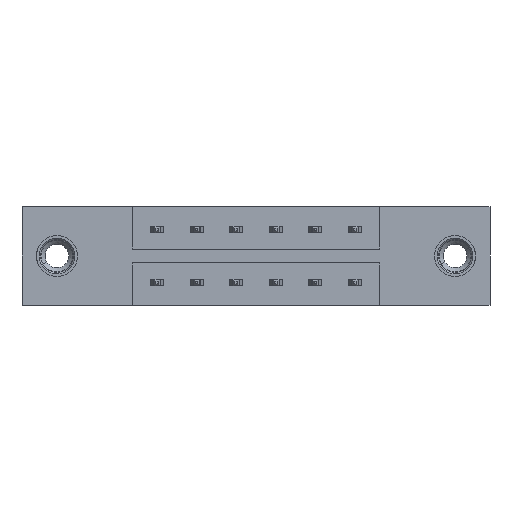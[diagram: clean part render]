
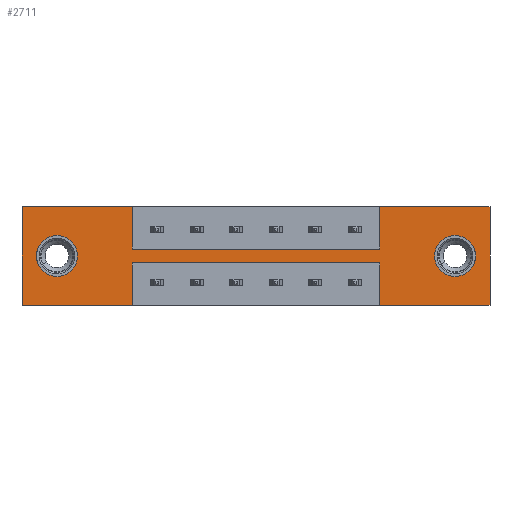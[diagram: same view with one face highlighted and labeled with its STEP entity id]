
A CAD part, front view. The second image highlights one B-rep face of the part: STEP entity #2711.
In plain terms, the highlighted planar face has unit normal (0, -1, 0).
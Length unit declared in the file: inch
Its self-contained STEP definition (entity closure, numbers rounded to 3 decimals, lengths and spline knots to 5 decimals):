
#9 = ORIENTED_EDGE ( 'NONE', *, *, #3987, .F. ) ;
#28 = CARTESIAN_POINT ( 'NONE',  ( 0.1325, 0., -0.1095 ) ) ;
#43 = AXIS2_PLACEMENT_3D ( 'NONE', #4647, #4583, #858 ) ;
#75 = VERTEX_POINT ( 'NONE', #8183 ) ;
#105 = EDGE_CURVE ( 'NONE', #1922, #75, #3162, .T. ) ;
#159 = EDGE_CURVE ( 'NONE', #5463, #1922, #8088, .T. ) ;
#179 = DIRECTION ( 'NONE',  ( 0., 0., -1. ) ) ;
#241 = VERTEX_POINT ( 'NONE', #5210 ) ;
#253 = DIRECTION ( 'NONE',  ( 0., 0., -1. ) ) ;
#374 = VERTEX_POINT ( 'NONE', #9278 ) ;
#519 = LINE ( 'NONE', #8531, #4059 ) ;
#583 = DIRECTION ( 'NONE',  ( 0., 0., 1. ) ) ;
#628 = FACE_BOUND ( 'NONE', #6813, .T. ) ;
#663 = VECTOR ( 'NONE', #9193, 39.37008 ) ;
#706 = EDGE_LOOP ( 'NONE', ( #8567, #3923 ) ) ;
#814 = CARTESIAN_POINT ( 'NONE',  ( 1.3575, 0., -0.161 ) ) ;
#851 = CARTESIAN_POINT ( 'NONE',  ( 0., 0., -0.375 ) ) ;
#858 = DIRECTION ( 'NONE',  ( 0., 0., -1. ) ) ;
#913 = ORIENTED_EDGE ( 'NONE', *, *, #3880, .F. ) ;
#954 = EDGE_CURVE ( 'NONE', #241, #374, #7257, .T. ) ;
#984 = CARTESIAN_POINT ( 'NONE',  ( 0., 0., -0.375 ) ) ;
#1067 = ORIENTED_EDGE ( 'NONE', *, *, #5295, .T. ) ;
#1130 = VECTOR ( 'NONE', #2078, 39.37008 ) ;
#1239 = EDGE_CURVE ( 'NONE', #5102, #2460, #4670, .T. ) ;
#1309 = CARTESIAN_POINT ( 'NONE',  ( 0.4175, 0., -0.161 ) ) ;
#1341 = CARTESIAN_POINT ( 'NONE',  ( 0., 0., 0. ) ) ;
#1405 = DIRECTION ( 'NONE',  ( 0., 1., 0. ) ) ;
#1406 = VERTEX_POINT ( 'NONE', #3636 ) ;
#1630 = CARTESIAN_POINT ( 'NONE',  ( 1.6425, 0., -0.1875 ) ) ;
#1670 = EDGE_CURVE ( 'NONE', #1406, #6208, #9110, .T. ) ;
#1763 = DIRECTION ( 'NONE',  ( 0., 0., -1. ) ) ;
#1913 = VECTOR ( 'NONE', #2419, 39.37008 ) ;
#1922 = VERTEX_POINT ( 'NONE', #5045 ) ;
#2024 = LINE ( 'NONE', #1309, #6029 ) ;
#2039 = CARTESIAN_POINT ( 'NONE',  ( 0.4175, 0., -0.214 ) ) ;
#2078 = DIRECTION ( 'NONE',  ( 1., 0., 0. ) ) ;
#2124 = EDGE_CURVE ( 'NONE', #374, #241, #6973, .T. ) ;
#2221 = VECTOR ( 'NONE', #8911, 39.37008 ) ;
#2318 = DIRECTION ( 'NONE',  ( 0., 0., 1. ) ) ;
#2326 = LINE ( 'NONE', #5393, #3517 ) ;
#2419 = DIRECTION ( 'NONE',  ( 0., 0., 1. ) ) ;
#2433 = DIRECTION ( 'NONE',  ( 1., 0., 0. ) ) ;
#2460 = VERTEX_POINT ( 'NONE', #9529 ) ;
#2687 = CARTESIAN_POINT ( 'NONE',  ( 1.3575, 0., -0.161 ) ) ;
#2711 = ADVANCED_FACE ( 'NONE', ( #6384, #628, #5810 ), #6848, .T. ) ;
#2805 = EDGE_CURVE ( 'NONE', #6142, #5102, #4406, .T. ) ;
#2875 = CARTESIAN_POINT ( 'NONE',  ( 0.1325, 0., -0.1875 ) ) ;
#2885 = ORIENTED_EDGE ( 'NONE', *, *, #1239, .F. ) ;
#2954 = EDGE_CURVE ( 'NONE', #7374, #1406, #519, .T. ) ;
#3088 = DIRECTION ( 'NONE',  ( 0., -1., 0. ) ) ;
#3132 = EDGE_CURVE ( 'NONE', #2460, #4090, #2024, .T. ) ;
#3162 = LINE ( 'NONE', #9605, #2221 ) ;
#3517 = VECTOR ( 'NONE', #2433, 39.37008 ) ;
#3620 = CIRCLE ( 'NONE', #6883, 0.078 ) ;
#3636 = CARTESIAN_POINT ( 'NONE',  ( 1.775, 0., -0.375 ) ) ;
#3832 = CARTESIAN_POINT ( 'NONE',  ( 1.775, 0., 0. ) ) ;
#3880 = EDGE_CURVE ( 'NONE', #6208, #5463, #4092, .T. ) ;
#3923 = ORIENTED_EDGE ( 'NONE', *, *, #2124, .T. ) ;
#3987 = EDGE_CURVE ( 'NONE', #75, #6142, #4557, .T. ) ;
#4059 = VECTOR ( 'NONE', #1763, 39.37008 ) ;
#4090 = VERTEX_POINT ( 'NONE', #4901 ) ;
#4092 = LINE ( 'NONE', #8894, #7470 ) ;
#4104 = VERTEX_POINT ( 'NONE', #2687 ) ;
#4259 = ORIENTED_EDGE ( 'NONE', *, *, #2954, .F. ) ;
#4289 = ORIENTED_EDGE ( 'NONE', *, *, #2805, .F. ) ;
#4406 = LINE ( 'NONE', #8373, #1913 ) ;
#4555 = EDGE_LOOP ( 'NONE', ( #913, #6363, #4259, #5035, #7524, #6803, #5549, #2885, #4289, #9, #8755, #8306 ) ) ;
#4557 = LINE ( 'NONE', #984, #663 ) ;
#4583 = DIRECTION ( 'NONE',  ( 0., 1., 0. ) ) ;
#4647 = CARTESIAN_POINT ( 'NONE',  ( 1.6425, 0., -0.1875 ) ) ;
#4653 = CARTESIAN_POINT ( 'NONE',  ( 1.3575, 0., -0.375 ) ) ;
#4670 = LINE ( 'NONE', #1341, #1130 ) ;
#4729 = VERTEX_POINT ( 'NONE', #28 ) ;
#4767 = DIRECTION ( 'NONE',  ( 0., 1., 0. ) ) ;
#4894 = CARTESIAN_POINT ( 'NONE',  ( 0., 0., -0.375 ) ) ;
#4901 = CARTESIAN_POINT ( 'NONE',  ( 0.4175, 0., -0.161 ) ) ;
#4979 = CARTESIAN_POINT ( 'NONE',  ( 0., 0., 0. ) ) ;
#5000 = DIRECTION ( 'NONE',  ( 0., 1., 0. ) ) ;
#5035 = ORIENTED_EDGE ( 'NONE', *, *, #5104, .F. ) ;
#5045 = CARTESIAN_POINT ( 'NONE',  ( 0.4175, 0., -0.214 ) ) ;
#5102 = VERTEX_POINT ( 'NONE', #4979 ) ;
#5104 = EDGE_CURVE ( 'NONE', #6469, #7374, #9489, .T. ) ;
#5210 = CARTESIAN_POINT ( 'NONE',  ( 1.6425, 0., -0.1095 ) ) ;
#5295 = EDGE_CURVE ( 'NONE', #4729, #8133, #3620, .T. ) ;
#5393 = CARTESIAN_POINT ( 'NONE',  ( 0.4175, 0., -0.161 ) ) ;
#5463 = VERTEX_POINT ( 'NONE', #8370 ) ;
#5501 = VECTOR ( 'NONE', #7284, 39.37008 ) ;
#5549 = ORIENTED_EDGE ( 'NONE', *, *, #3132, .F. ) ;
#5810 = FACE_OUTER_BOUND ( 'NONE', #4555, .T. ) ;
#6029 = VECTOR ( 'NONE', #7369, 39.37008 ) ;
#6072 = LINE ( 'NONE', #814, #6437 ) ;
#6142 = VERTEX_POINT ( 'NONE', #4894 ) ;
#6208 = VERTEX_POINT ( 'NONE', #4653 ) ;
#6363 = ORIENTED_EDGE ( 'NONE', *, *, #1670, .F. ) ;
#6384 = FACE_BOUND ( 'NONE', #706, .T. ) ;
#6437 = VECTOR ( 'NONE', #2318, 39.37008 ) ;
#6469 = VERTEX_POINT ( 'NONE', #8650 ) ;
#6643 = DIRECTION ( 'NONE',  ( -1., 0., 0. ) ) ;
#6648 = ORIENTED_EDGE ( 'NONE', *, *, #8028, .T. ) ;
#6769 = AXIS2_PLACEMENT_3D ( 'NONE', #2875, #5000, #583 ) ;
#6803 = ORIENTED_EDGE ( 'NONE', *, *, #9226, .F. ) ;
#6813 = EDGE_LOOP ( 'NONE', ( #1067, #6648 ) ) ;
#6848 = PLANE ( 'NONE',  #8982 ) ;
#6883 = AXIS2_PLACEMENT_3D ( 'NONE', #8143, #1405, #8065 ) ;
#6907 = CIRCLE ( 'NONE', #6769, 0.078 ) ;
#6973 = CIRCLE ( 'NONE', #43, 0.078 ) ;
#7114 = AXIS2_PLACEMENT_3D ( 'NONE', #1630, #4767, #253 ) ;
#7257 = CIRCLE ( 'NONE', #7114, 0.078 ) ;
#7284 = DIRECTION ( 'NONE',  ( 1., 0., 0. ) ) ;
#7369 = DIRECTION ( 'NONE',  ( 0., 0., -1. ) ) ;
#7374 = VERTEX_POINT ( 'NONE', #3832 ) ;
#7416 = DIRECTION ( 'NONE',  ( 0., 0., 1. ) ) ;
#7439 = CARTESIAN_POINT ( 'NONE',  ( 0.1325, 0., -0.2655 ) ) ;
#7470 = VECTOR ( 'NONE', #7416, 39.37008 ) ;
#7524 = ORIENTED_EDGE ( 'NONE', *, *, #9475, .F. ) ;
#7622 = VECTOR ( 'NONE', #6643, 39.37008 ) ;
#8028 = EDGE_CURVE ( 'NONE', #8133, #4729, #6907, .T. ) ;
#8065 = DIRECTION ( 'NONE',  ( 0., 0., 1. ) ) ;
#8088 = LINE ( 'NONE', #2039, #7622 ) ;
#8133 = VERTEX_POINT ( 'NONE', #7439 ) ;
#8143 = CARTESIAN_POINT ( 'NONE',  ( 0.1325, 0., -0.1875 ) ) ;
#8165 = VECTOR ( 'NONE', #8418, 39.37008 ) ;
#8183 = CARTESIAN_POINT ( 'NONE',  ( 0.4175, 0., -0.375 ) ) ;
#8306 = ORIENTED_EDGE ( 'NONE', *, *, #159, .F. ) ;
#8370 = CARTESIAN_POINT ( 'NONE',  ( 1.3575, 0., -0.214 ) ) ;
#8373 = CARTESIAN_POINT ( 'NONE',  ( 0., 0., 0. ) ) ;
#8418 = DIRECTION ( 'NONE',  ( -1., 0., 0. ) ) ;
#8531 = CARTESIAN_POINT ( 'NONE',  ( 1.775, 0., 0. ) ) ;
#8554 = CARTESIAN_POINT ( 'NONE',  ( 0., 0., -0.375 ) ) ;
#8567 = ORIENTED_EDGE ( 'NONE', *, *, #954, .T. ) ;
#8650 = CARTESIAN_POINT ( 'NONE',  ( 1.3575, 0., 0. ) ) ;
#8755 = ORIENTED_EDGE ( 'NONE', *, *, #105, .F. ) ;
#8767 = CARTESIAN_POINT ( 'NONE',  ( 0., 0., 0. ) ) ;
#8894 = CARTESIAN_POINT ( 'NONE',  ( 1.3575, 0., -0.214 ) ) ;
#8911 = DIRECTION ( 'NONE',  ( 0., 0., -1. ) ) ;
#8982 = AXIS2_PLACEMENT_3D ( 'NONE', #851, #3088, #179 ) ;
#9110 = LINE ( 'NONE', #8554, #8165 ) ;
#9193 = DIRECTION ( 'NONE',  ( -1., 0., 0. ) ) ;
#9226 = EDGE_CURVE ( 'NONE', #4090, #4104, #2326, .T. ) ;
#9278 = CARTESIAN_POINT ( 'NONE',  ( 1.6425, 0., -0.2655 ) ) ;
#9475 = EDGE_CURVE ( 'NONE', #4104, #6469, #6072, .T. ) ;
#9489 = LINE ( 'NONE', #8767, #5501 ) ;
#9529 = CARTESIAN_POINT ( 'NONE',  ( 0.4175, 0., 0. ) ) ;
#9605 = CARTESIAN_POINT ( 'NONE',  ( 0.4175, 0., -0.214 ) ) ;
